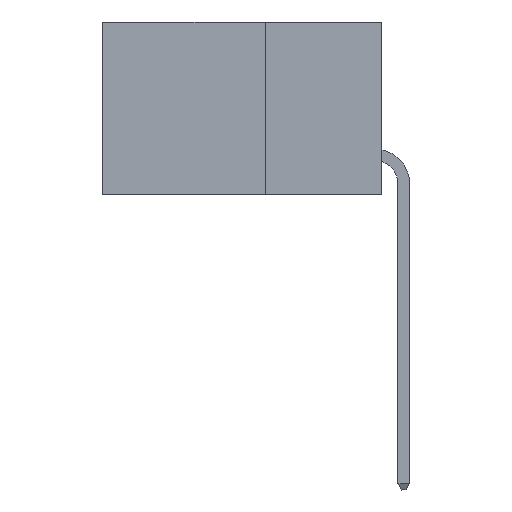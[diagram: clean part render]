
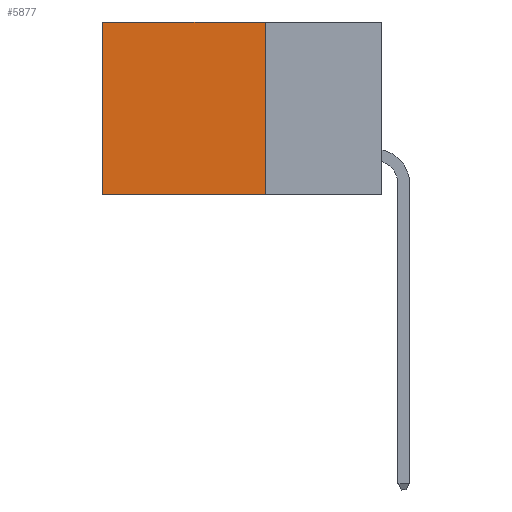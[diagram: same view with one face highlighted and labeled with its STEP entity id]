
A CAD part, left-side view. The second image highlights one B-rep face of the part: STEP entity #5877.
In plain terms, the highlighted planar face has unit normal (-1, 0, 0).
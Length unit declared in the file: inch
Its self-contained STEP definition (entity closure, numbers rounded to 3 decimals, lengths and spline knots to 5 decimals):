
#56 = DIRECTION ( 'NONE',  ( 0., 1., 0. ) ) ;
#581 = FACE_OUTER_BOUND ( 'NONE', #2042, .T. ) ;
#903 = DIRECTION ( 'NONE',  ( 1., 0., 0. ) ) ;
#1348 = CARTESIAN_POINT ( 'NONE',  ( 0.2875, 0.25, -0.37 ) ) ;
#2042 = EDGE_LOOP ( 'NONE', ( #9294, #9298, #9331, #9341 ) ) ;
#2908 = CARTESIAN_POINT ( 'NONE',  ( 0.2875, 0.6, -0.37 ) ) ;
#3282 = EDGE_CURVE ( 'NONE', #10337, #7939, #11797, .T. ) ;
#3495 = AXIS2_PLACEMENT_3D ( 'NONE', #13473, #903, #8781 ) ;
#3691 = CARTESIAN_POINT ( 'NONE',  ( 0.2875, 0.25, 0. ) ) ;
#5201 = VECTOR ( 'NONE', #56, 39.37008 ) ;
#5322 = LINE ( 'NONE', #3691, #7758 ) ;
#5372 = EDGE_CURVE ( 'NONE', #11903, #5722, #5322, .T. ) ;
#5641 = CARTESIAN_POINT ( 'NONE',  ( 0.2875, 0.25, 0. ) ) ;
#5722 = VERTEX_POINT ( 'NONE', #7509 ) ;
#5877 = ADVANCED_FACE ( 'NONE', ( #581 ), #6709, .F. ) ;
#6495 = VECTOR ( 'NONE', #10955, 39.37008 ) ;
#6674 = LINE ( 'NONE', #7289, #11672 ) ;
#6709 = PLANE ( 'NONE',  #3495 ) ;
#7289 = CARTESIAN_POINT ( 'NONE',  ( 0.2875, 0.25, 0. ) ) ;
#7509 = CARTESIAN_POINT ( 'NONE',  ( 0.2875, 0.25, -0.37 ) ) ;
#7758 = VECTOR ( 'NONE', #12820, 39.37008 ) ;
#7939 = VERTEX_POINT ( 'NONE', #2908 ) ;
#8781 = DIRECTION ( 'NONE',  ( 0., 0., -1. ) ) ;
#9294 = ORIENTED_EDGE ( 'NONE', *, *, #3282, .T. ) ;
#9298 = ORIENTED_EDGE ( 'NONE', *, *, #9379, .F. ) ;
#9331 = ORIENTED_EDGE ( 'NONE', *, *, #5372, .F. ) ;
#9341 = ORIENTED_EDGE ( 'NONE', *, *, #10947, .T. ) ;
#9379 = EDGE_CURVE ( 'NONE', #5722, #7939, #10988, .T. ) ;
#10313 = CARTESIAN_POINT ( 'NONE',  ( 0.2875, 0.6, 0. ) ) ;
#10337 = VERTEX_POINT ( 'NONE', #10313 ) ;
#10795 = CARTESIAN_POINT ( 'NONE',  ( 0.2875, 0.6, 0. ) ) ;
#10947 = EDGE_CURVE ( 'NONE', #11903, #10337, #6674, .T. ) ;
#10955 = DIRECTION ( 'NONE',  ( 0., 0., -1. ) ) ;
#10988 = LINE ( 'NONE', #1348, #5201 ) ;
#11672 = VECTOR ( 'NONE', #12152, 39.37008 ) ;
#11797 = LINE ( 'NONE', #10795, #6495 ) ;
#11903 = VERTEX_POINT ( 'NONE', #5641 ) ;
#12152 = DIRECTION ( 'NONE',  ( 0., 1., 0. ) ) ;
#12820 = DIRECTION ( 'NONE',  ( 0., 0., -1. ) ) ;
#13473 = CARTESIAN_POINT ( 'NONE',  ( 0.2875, 0.25, 0. ) ) ;
